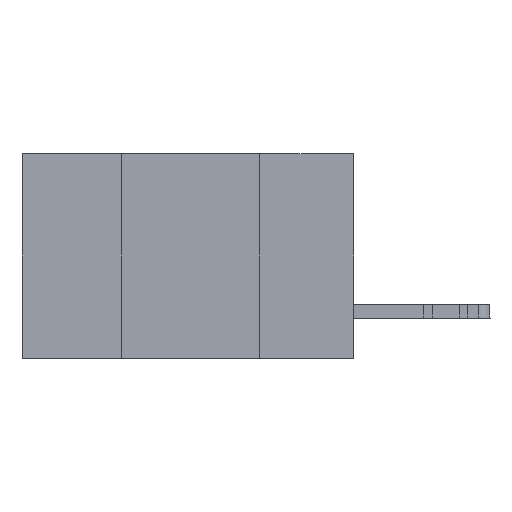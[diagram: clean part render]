
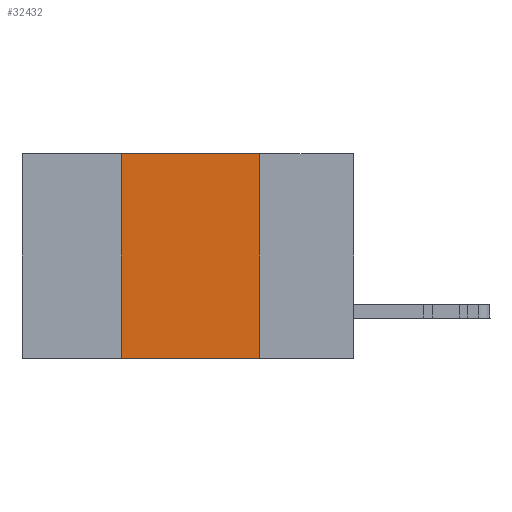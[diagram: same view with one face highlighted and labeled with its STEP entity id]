
A CAD part, left-side view. The second image highlights one B-rep face of the part: STEP entity #32432.
In plain terms, the highlighted planar face has unit normal (-1, 0, 0).
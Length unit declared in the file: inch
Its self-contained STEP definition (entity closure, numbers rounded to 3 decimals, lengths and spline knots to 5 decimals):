
#2160 = ORIENTED_EDGE ( 'NONE', *, *, #35997, .F. ) ;
#4181 = CARTESIAN_POINT ( 'NONE',  ( 0., 0.6, 0. ) ) ;
#4276 = CARTESIAN_POINT ( 'NONE',  ( 0., 0.42, 0. ) ) ;
#6653 = AXIS2_PLACEMENT_3D ( 'NONE', #4181, #18694, #29614 ) ;
#7413 = CARTESIAN_POINT ( 'NONE',  ( 0., 0.17, -0.37 ) ) ;
#9010 = VERTEX_POINT ( 'NONE', #43909 ) ;
#9572 = CARTESIAN_POINT ( 'NONE',  ( 0., 0.17, 0. ) ) ;
#12101 = VECTOR ( 'NONE', #36465, 39.37008 ) ;
#14677 = DIRECTION ( 'NONE',  ( 0., 0., -1. ) ) ;
#14931 = VERTEX_POINT ( 'NONE', #9572 ) ;
#15290 = VECTOR ( 'NONE', #14677, 39.37008 ) ;
#16222 = VECTOR ( 'NONE', #18436, 39.37008 ) ;
#18436 = DIRECTION ( 'NONE',  ( 0., -1., 0. ) ) ;
#18694 = DIRECTION ( 'NONE',  ( 1., 0., 0. ) ) ;
#19005 = PLANE ( 'NONE',  #6653 ) ;
#19777 = LINE ( 'NONE', #45864, #37723 ) ;
#20315 = EDGE_CURVE ( 'NONE', #44043, #22397, #46111, .T. ) ;
#22397 = VERTEX_POINT ( 'NONE', #7413 ) ;
#22991 = EDGE_CURVE ( 'NONE', #14931, #22397, #29250, .T. ) ;
#23051 = EDGE_CURVE ( 'NONE', #9010, #14931, #19777, .T. ) ;
#25018 = CARTESIAN_POINT ( 'NONE',  ( 0., 0.17, 0. ) ) ;
#25772 = FACE_OUTER_BOUND ( 'NONE', #30353, .T. ) ;
#26273 = ORIENTED_EDGE ( 'NONE', *, *, #20315, .T. ) ;
#27137 = ORIENTED_EDGE ( 'NONE', *, *, #23051, .F. ) ;
#28207 = ORIENTED_EDGE ( 'NONE', *, *, #22991, .F. ) ;
#29250 = LINE ( 'NONE', #25018, #15290 ) ;
#29614 = DIRECTION ( 'NONE',  ( 0., 0., -1. ) ) ;
#30353 = EDGE_LOOP ( 'NONE', ( #28207, #27137, #2160, #26273 ) ) ;
#32432 = ADVANCED_FACE ( 'NONE', ( #25772 ), #19005, .F. ) ;
#33098 = CARTESIAN_POINT ( 'NONE',  ( 0., 0.42, -0.37 ) ) ;
#34708 = DIRECTION ( 'NONE',  ( 0., -1., 0. ) ) ;
#35997 = EDGE_CURVE ( 'NONE', #44043, #9010, #38992, .T. ) ;
#36465 = DIRECTION ( 'NONE',  ( 0., 0., 1. ) ) ;
#36594 = CARTESIAN_POINT ( 'NONE',  ( 0., 0.6, -0.37 ) ) ;
#37723 = VECTOR ( 'NONE', #34708, 39.37008 ) ;
#38992 = LINE ( 'NONE', #4276, #12101 ) ;
#43909 = CARTESIAN_POINT ( 'NONE',  ( 0., 0.42, 0. ) ) ;
#44043 = VERTEX_POINT ( 'NONE', #33098 ) ;
#45864 = CARTESIAN_POINT ( 'NONE',  ( 0., 0.6, 0. ) ) ;
#46111 = LINE ( 'NONE', #36594, #16222 ) ;
